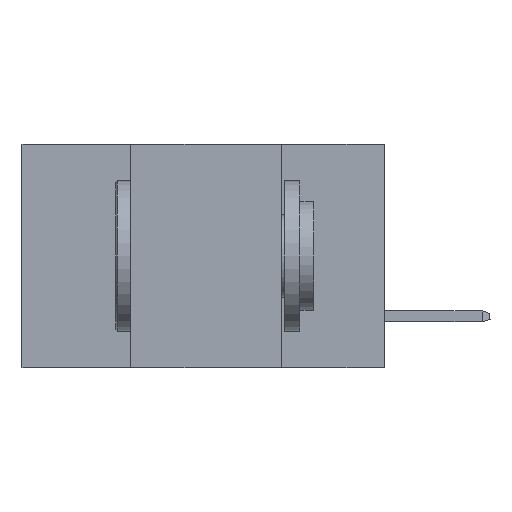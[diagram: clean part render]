
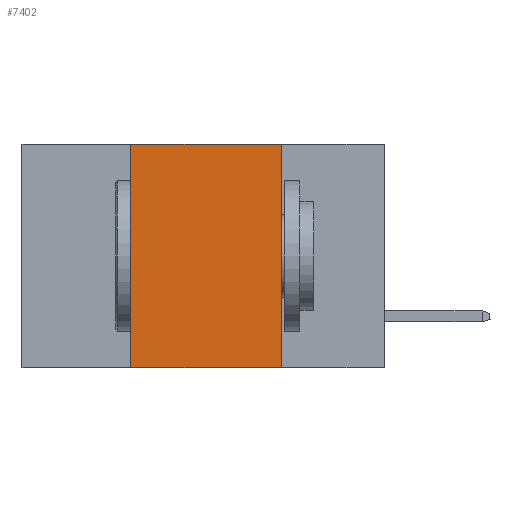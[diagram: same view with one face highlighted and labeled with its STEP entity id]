
A CAD part, left-side view. The second image highlights one B-rep face of the part: STEP entity #7402.
In plain terms, the highlighted planar face has unit normal (-1, 0, 0).
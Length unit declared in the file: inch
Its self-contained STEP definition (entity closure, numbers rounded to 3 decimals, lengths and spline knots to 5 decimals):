
#2367 = EDGE_LOOP ( 'NONE', ( #7048, #14288, #2727, #18107 ) ) ;
#2727 = ORIENTED_EDGE ( 'NONE', *, *, #8082, .F. ) ;
#2879 = CARTESIAN_POINT ( 'NONE',  ( 0., 0.6, 0. ) ) ;
#3587 = CARTESIAN_POINT ( 'NONE',  ( 0., 0.42, 0. ) ) ;
#4968 = PLANE ( 'NONE',  #24933 ) ;
#6437 = VERTEX_POINT ( 'NONE', #19584 ) ;
#7028 = VECTOR ( 'NONE', #15312, 39.37008 ) ;
#7048 = ORIENTED_EDGE ( 'NONE', *, *, #11813, .F. ) ;
#7305 = CARTESIAN_POINT ( 'NONE',  ( 0., 0.6, 0. ) ) ;
#7402 = ADVANCED_FACE ( 'NONE', ( #21285 ), #4968, .F. ) ;
#8082 = EDGE_CURVE ( 'NONE', #6437, #29808, #13960, .T. ) ;
#9646 = DIRECTION ( 'NONE',  ( 0., 0., -1. ) ) ;
#9907 = CARTESIAN_POINT ( 'NONE',  ( 0., 0.17, -0.37 ) ) ;
#11107 = LINE ( 'NONE', #2879, #24581 ) ;
#11813 = EDGE_CURVE ( 'NONE', #16389, #21320, #27505, .T. ) ;
#12576 = EDGE_CURVE ( 'NONE', #6437, #21320, #14318, .T. ) ;
#13957 = VECTOR ( 'NONE', #23553, 39.37008 ) ;
#13960 = LINE ( 'NONE', #3587, #7028 ) ;
#14127 = CARTESIAN_POINT ( 'NONE',  ( 0., 0.17, 0. ) ) ;
#14288 = ORIENTED_EDGE ( 'NONE', *, *, #23365, .F. ) ;
#14318 = LINE ( 'NONE', #29647, #27835 ) ;
#15312 = DIRECTION ( 'NONE',  ( 0., 0., 1. ) ) ;
#16389 = VERTEX_POINT ( 'NONE', #14127 ) ;
#17677 = DIRECTION ( 'NONE',  ( 0., -1., 0. ) ) ;
#18107 = ORIENTED_EDGE ( 'NONE', *, *, #12576, .T. ) ;
#19584 = CARTESIAN_POINT ( 'NONE',  ( 0., 0.42, -0.37 ) ) ;
#21285 = FACE_OUTER_BOUND ( 'NONE', #2367, .T. ) ;
#21320 = VERTEX_POINT ( 'NONE', #9907 ) ;
#23365 = EDGE_CURVE ( 'NONE', #29808, #16389, #11107, .T. ) ;
#23553 = DIRECTION ( 'NONE',  ( 0., 0., -1. ) ) ;
#23597 = DIRECTION ( 'NONE',  ( 1., 0., 0. ) ) ;
#24581 = VECTOR ( 'NONE', #28311, 39.37008 ) ;
#24933 = AXIS2_PLACEMENT_3D ( 'NONE', #7305, #23597, #9646 ) ;
#25727 = CARTESIAN_POINT ( 'NONE',  ( 0., 0.17, 0. ) ) ;
#27505 = LINE ( 'NONE', #25727, #13957 ) ;
#27835 = VECTOR ( 'NONE', #17677, 39.37008 ) ;
#28311 = DIRECTION ( 'NONE',  ( 0., -1., 0. ) ) ;
#28334 = CARTESIAN_POINT ( 'NONE',  ( 0., 0.42, 0. ) ) ;
#29647 = CARTESIAN_POINT ( 'NONE',  ( 0., 0.6, -0.37 ) ) ;
#29808 = VERTEX_POINT ( 'NONE', #28334 ) ;
